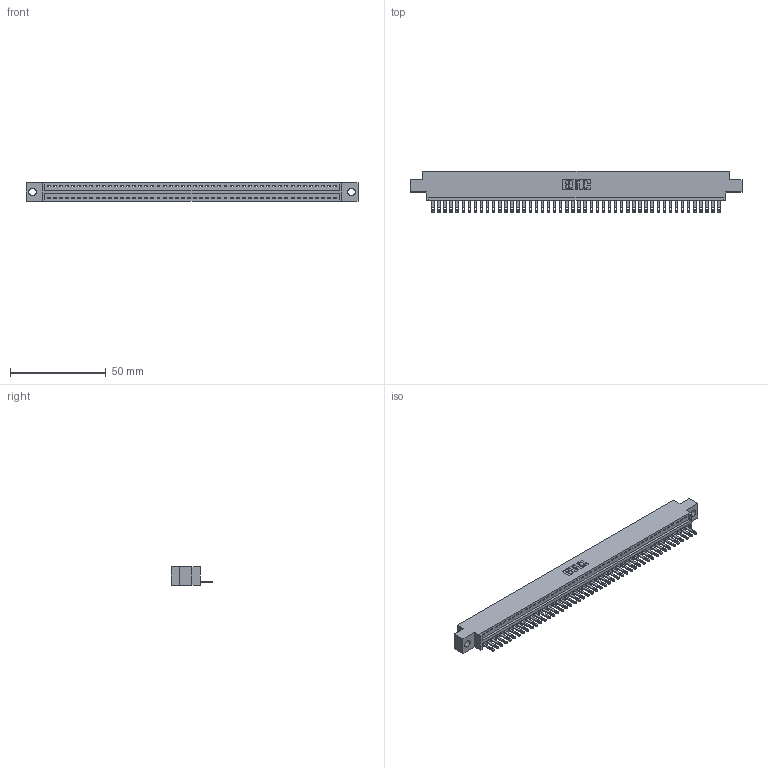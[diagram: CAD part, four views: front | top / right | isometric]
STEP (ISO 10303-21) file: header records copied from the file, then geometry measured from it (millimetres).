
FILE_DESCRIPTION (( 'STEP AP203' ), '1' );
FILE_NAME ('346-048-500-604.STEP', '2022-05-09T22:47:40', ( '' ), ( '' ), 'SwSTEP 2.0', 'SolidWorks 2020', '' );
FILE_SCHEMA (( 'CONFIG_CONTROL_DESIGN' ));
Length unit declared in the file: inch
Products named in the file (3): 346 Part_0.170 Offset - 0.156 Dia-TH; 346-048-500-604; 345-292-001_345-293-100
Assembly tree (49 placements, depth 2):
  346-048-500-604
    346 Part_0.170 Offset - 0.156 Dia-TH
    345-292-001_345-293-100  x48
Bounding box: 172.97 x 21.84 x 9.4 mm (x, y, z)
Volume: 16367.9 mm3; surface area: 20632 mm2
Topology: 49 solids, 49 shells, 2732 faces, 8441 edges, 5626 vertices
Faces by surface type: plane 1726, cylinder 1006
Entity records: 29463 total; most frequent: CARTESIAN_POINT 5058, ORIENTED_EDGE 5038, DIRECTION 4455, EDGE_CURVE 2519, VECTOR 2191, LINE 2191, VERTEX_POINT 1678, AXIS2_PLACEMENT_3D 1132
